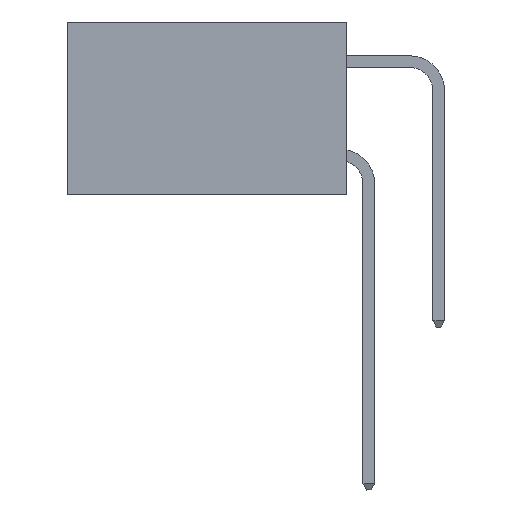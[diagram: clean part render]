
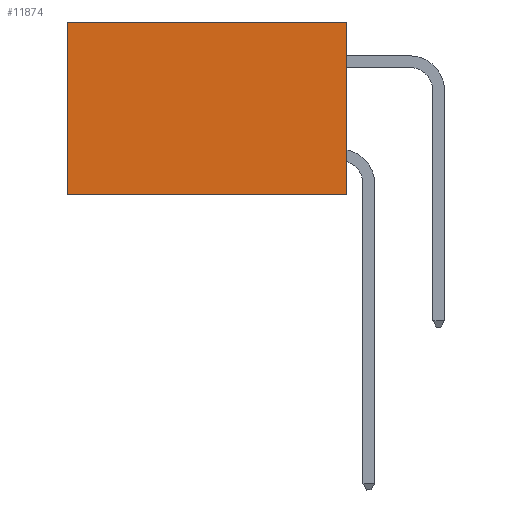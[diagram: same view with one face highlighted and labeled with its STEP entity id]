
A CAD part, left-side view. The second image highlights one B-rep face of the part: STEP entity #11874.
In plain terms, the highlighted planar face has unit normal (-1, 0, 0).
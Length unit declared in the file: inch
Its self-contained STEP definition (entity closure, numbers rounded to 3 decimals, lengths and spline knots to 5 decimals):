
#117 = VECTOR ( 'NONE', #25420, 39.37008 ) ;
#929 = EDGE_LOOP ( 'NONE', ( #20700, #12361, #18023, #12374 ) ) ;
#1448 = DIRECTION ( 'NONE',  ( 0., 0., -1. ) ) ;
#2452 = DIRECTION ( 'NONE',  ( 0., 0., -1. ) ) ;
#2648 = EDGE_CURVE ( 'NONE', #22845, #9985, #19784, .T. ) ;
#3094 = CARTESIAN_POINT ( 'NONE',  ( 0.2875, 0., 0. ) ) ;
#3915 = PLANE ( 'NONE',  #14487 ) ;
#5346 = CARTESIAN_POINT ( 'NONE',  ( 0.2875, 0.6, 0. ) ) ;
#6708 = CARTESIAN_POINT ( 'NONE',  ( 0.2875, 0.6, 0. ) ) ;
#7253 = CARTESIAN_POINT ( 'NONE',  ( 0.2875, 0., -0.37 ) ) ;
#7925 = EDGE_CURVE ( 'NONE', #22845, #15580, #26950, .T. ) ;
#7971 = EDGE_CURVE ( 'NONE', #15580, #14712, #22147, .T. ) ;
#8433 = DIRECTION ( 'NONE',  ( 0., 1., 0. ) ) ;
#9740 = CARTESIAN_POINT ( 'NONE',  ( 0.2875, 0., 0. ) ) ;
#9985 = VERTEX_POINT ( 'NONE', #7253 ) ;
#10578 = DIRECTION ( 'NONE',  ( 1., 0., 0. ) ) ;
#11874 = ADVANCED_FACE ( 'NONE', ( #28358 ), #3915, .F. ) ;
#12361 = ORIENTED_EDGE ( 'NONE', *, *, #16458, .F. ) ;
#12374 = ORIENTED_EDGE ( 'NONE', *, *, #7925, .T. ) ;
#13525 = DIRECTION ( 'NONE',  ( 0., 1., 0. ) ) ;
#14487 = AXIS2_PLACEMENT_3D ( 'NONE', #14595, #10578, #1448 ) ;
#14560 = VECTOR ( 'NONE', #8433, 39.37008 ) ;
#14595 = CARTESIAN_POINT ( 'NONE',  ( 0.2875, 0., 0. ) ) ;
#14712 = VERTEX_POINT ( 'NONE', #15946 ) ;
#15580 = VERTEX_POINT ( 'NONE', #5346 ) ;
#15946 = CARTESIAN_POINT ( 'NONE',  ( 0.2875, 0.6, -0.37 ) ) ;
#16458 = EDGE_CURVE ( 'NONE', #9985, #14712, #27370, .T. ) ;
#17709 = VECTOR ( 'NONE', #2452, 39.37008 ) ;
#18023 = ORIENTED_EDGE ( 'NONE', *, *, #2648, .F. ) ;
#18091 = VECTOR ( 'NONE', #13525, 39.37008 ) ;
#19784 = LINE ( 'NONE', #3094, #117 ) ;
#20700 = ORIENTED_EDGE ( 'NONE', *, *, #7971, .T. ) ;
#22147 = LINE ( 'NONE', #6708, #17709 ) ;
#22845 = VERTEX_POINT ( 'NONE', #9740 ) ;
#24330 = CARTESIAN_POINT ( 'NONE',  ( 0.2875, 0., -0.37 ) ) ;
#25420 = DIRECTION ( 'NONE',  ( 0., 0., -1. ) ) ;
#26950 = LINE ( 'NONE', #28354, #14560 ) ;
#27370 = LINE ( 'NONE', #24330, #18091 ) ;
#28354 = CARTESIAN_POINT ( 'NONE',  ( 0.2875, 0., 0. ) ) ;
#28358 = FACE_OUTER_BOUND ( 'NONE', #929, .T. ) ;
